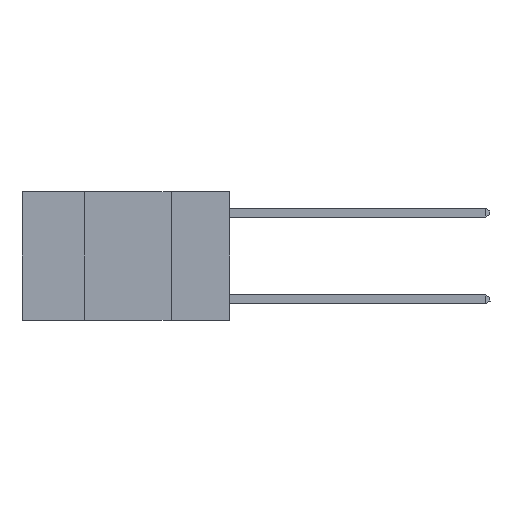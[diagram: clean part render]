
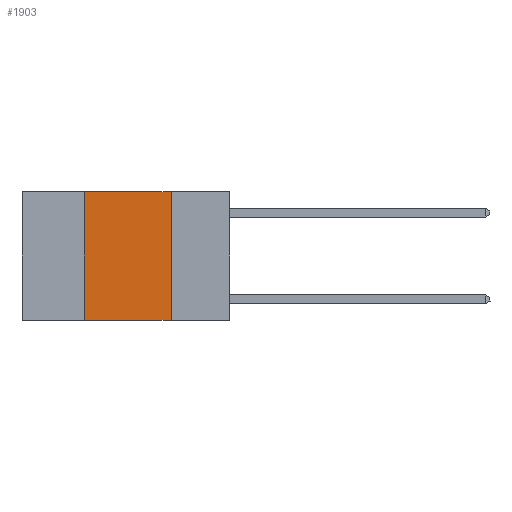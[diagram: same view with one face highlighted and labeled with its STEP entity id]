
A CAD part, left-side view. The second image highlights one B-rep face of the part: STEP entity #1903.
In plain terms, the highlighted planar face has unit normal (-1, 0, 0).
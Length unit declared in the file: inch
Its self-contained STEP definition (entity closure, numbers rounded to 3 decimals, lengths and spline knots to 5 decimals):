
#125 = VECTOR ( 'NONE', #3851, 39.37008 ) ;
#794 = CARTESIAN_POINT ( 'NONE',  ( 0., 0.17, 0. ) ) ;
#1777 = CARTESIAN_POINT ( 'NONE',  ( 0., 0.6, 0. ) ) ;
#1841 = VECTOR ( 'NONE', #3882, 39.37008 ) ;
#1864 = CARTESIAN_POINT ( 'NONE',  ( 0., 0.6, -0.37 ) ) ;
#1903 = ADVANCED_FACE ( 'NONE', ( #6909 ), #5638, .F. ) ;
#2246 = DIRECTION ( 'NONE',  ( 0., -1., 0. ) ) ;
#2787 = CARTESIAN_POINT ( 'NONE',  ( 0., 0.42, -0.37 ) ) ;
#3119 = EDGE_CURVE ( 'NONE', #4329, #7998, #4331, .T. ) ;
#3260 = EDGE_CURVE ( 'NONE', #4329, #9989, #4477, .T. ) ;
#3268 = VERTEX_POINT ( 'NONE', #9960 ) ;
#3851 = DIRECTION ( 'NONE',  ( 0., 0., -1. ) ) ;
#3882 = DIRECTION ( 'NONE',  ( 0., -1., 0. ) ) ;
#4032 = VECTOR ( 'NONE', #6354, 39.37008 ) ;
#4329 = VERTEX_POINT ( 'NONE', #2787 ) ;
#4331 = LINE ( 'NONE', #8031, #4032 ) ;
#4477 = LINE ( 'NONE', #1864, #1841 ) ;
#4750 = DIRECTION ( 'NONE',  ( 1., 0., 0. ) ) ;
#5081 = ORIENTED_EDGE ( 'NONE', *, *, #3119, .F. ) ;
#5638 = PLANE ( 'NONE',  #11421 ) ;
#5739 = LINE ( 'NONE', #8608, #7519 ) ;
#6354 = DIRECTION ( 'NONE',  ( 0., 0., 1. ) ) ;
#6909 = FACE_OUTER_BOUND ( 'NONE', #7512, .T. ) ;
#6917 = EDGE_CURVE ( 'NONE', #7998, #3268, #5739, .T. ) ;
#7512 = EDGE_LOOP ( 'NONE', ( #11726, #9477, #5081, #9537 ) ) ;
#7519 = VECTOR ( 'NONE', #2246, 39.37008 ) ;
#7750 = LINE ( 'NONE', #794, #125 ) ;
#7998 = VERTEX_POINT ( 'NONE', #11130 ) ;
#8031 = CARTESIAN_POINT ( 'NONE',  ( 0., 0.42, 0. ) ) ;
#8248 = CARTESIAN_POINT ( 'NONE',  ( 0., 0.17, -0.37 ) ) ;
#8608 = CARTESIAN_POINT ( 'NONE',  ( 0., 0.6, 0. ) ) ;
#9477 = ORIENTED_EDGE ( 'NONE', *, *, #6917, .F. ) ;
#9537 = ORIENTED_EDGE ( 'NONE', *, *, #3260, .T. ) ;
#9960 = CARTESIAN_POINT ( 'NONE',  ( 0., 0.17, 0. ) ) ;
#9989 = VERTEX_POINT ( 'NONE', #8248 ) ;
#10100 = EDGE_CURVE ( 'NONE', #3268, #9989, #7750, .T. ) ;
#10744 = DIRECTION ( 'NONE',  ( 0., 0., -1. ) ) ;
#11130 = CARTESIAN_POINT ( 'NONE',  ( 0., 0.42, 0. ) ) ;
#11421 = AXIS2_PLACEMENT_3D ( 'NONE', #1777, #4750, #10744 ) ;
#11726 = ORIENTED_EDGE ( 'NONE', *, *, #10100, .F. ) ;
